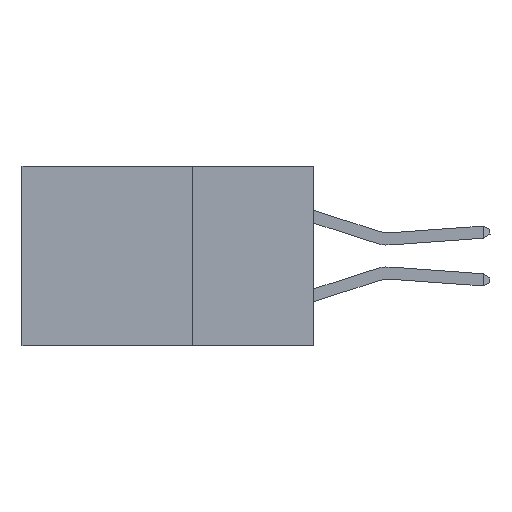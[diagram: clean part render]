
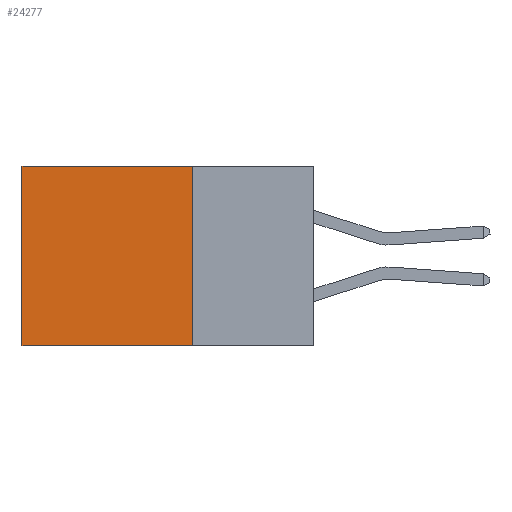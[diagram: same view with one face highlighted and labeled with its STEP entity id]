
A CAD part, left-side view. The second image highlights one B-rep face of the part: STEP entity #24277.
In plain terms, the highlighted planar face has unit normal (-1, 0, 0).
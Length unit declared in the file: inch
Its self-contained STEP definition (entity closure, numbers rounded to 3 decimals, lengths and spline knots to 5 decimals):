
#66 = CARTESIAN_POINT ( 'NONE',  ( 0.2875, 0.6, 0. ) ) ;
#115 = LINE ( 'NONE', #37844, #30173 ) ;
#186 = VERTEX_POINT ( 'NONE', #14894 ) ;
#1435 = DIRECTION ( 'NONE',  ( 0., 1., 0. ) ) ;
#1467 = ORIENTED_EDGE ( 'NONE', *, *, #35948, .F. ) ;
#2400 = VERTEX_POINT ( 'NONE', #36354 ) ;
#3860 = VECTOR ( 'NONE', #1435, 39.37008 ) ;
#3927 = EDGE_CURVE ( 'NONE', #186, #33715, #7591, .T. ) ;
#5180 = CARTESIAN_POINT ( 'NONE',  ( 0.2875, 0.25, -0.37 ) ) ;
#5795 = ORIENTED_EDGE ( 'NONE', *, *, #27406, .F. ) ;
#6362 = DIRECTION ( 'NONE',  ( 1., 0., 0. ) ) ;
#7448 = ORIENTED_EDGE ( 'NONE', *, *, #27264, .T. ) ;
#7591 = LINE ( 'NONE', #66, #30577 ) ;
#8667 = CARTESIAN_POINT ( 'NONE',  ( 0.2875, 0.6, -0.37 ) ) ;
#9277 = CARTESIAN_POINT ( 'NONE',  ( 0.2875, 0.25, 0. ) ) ;
#11930 = LINE ( 'NONE', #31369, #3860 ) ;
#13857 = AXIS2_PLACEMENT_3D ( 'NONE', #9277, #6362, #27329 ) ;
#14894 = CARTESIAN_POINT ( 'NONE',  ( 0.2875, 0.6, 0. ) ) ;
#21299 = ORIENTED_EDGE ( 'NONE', *, *, #3927, .T. ) ;
#23093 = DIRECTION ( 'NONE',  ( 0., 0., -1. ) ) ;
#23147 = DIRECTION ( 'NONE',  ( 0., 1., 0. ) ) ;
#24084 = DIRECTION ( 'NONE',  ( 0., 0., -1. ) ) ;
#24277 = ADVANCED_FACE ( 'NONE', ( #37412 ), #24306, .F. ) ;
#24306 = PLANE ( 'NONE',  #13857 ) ;
#25418 = VECTOR ( 'NONE', #23147, 39.37008 ) ;
#27264 = EDGE_CURVE ( 'NONE', #37464, #186, #11930, .T. ) ;
#27316 = LINE ( 'NONE', #5180, #25418 ) ;
#27329 = DIRECTION ( 'NONE',  ( 0., 0., -1. ) ) ;
#27406 = EDGE_CURVE ( 'NONE', #37464, #2400, #115, .T. ) ;
#30173 = VECTOR ( 'NONE', #23093, 39.37008 ) ;
#30577 = VECTOR ( 'NONE', #24084, 39.37008 ) ;
#31369 = CARTESIAN_POINT ( 'NONE',  ( 0.2875, 0.25, 0. ) ) ;
#32264 = EDGE_LOOP ( 'NONE', ( #21299, #1467, #5795, #7448 ) ) ;
#32999 = CARTESIAN_POINT ( 'NONE',  ( 0.2875, 0.25, 0. ) ) ;
#33715 = VERTEX_POINT ( 'NONE', #8667 ) ;
#35948 = EDGE_CURVE ( 'NONE', #2400, #33715, #27316, .T. ) ;
#36354 = CARTESIAN_POINT ( 'NONE',  ( 0.2875, 0.25, -0.37 ) ) ;
#37412 = FACE_OUTER_BOUND ( 'NONE', #32264, .T. ) ;
#37464 = VERTEX_POINT ( 'NONE', #32999 ) ;
#37844 = CARTESIAN_POINT ( 'NONE',  ( 0.2875, 0.25, 0. ) ) ;
